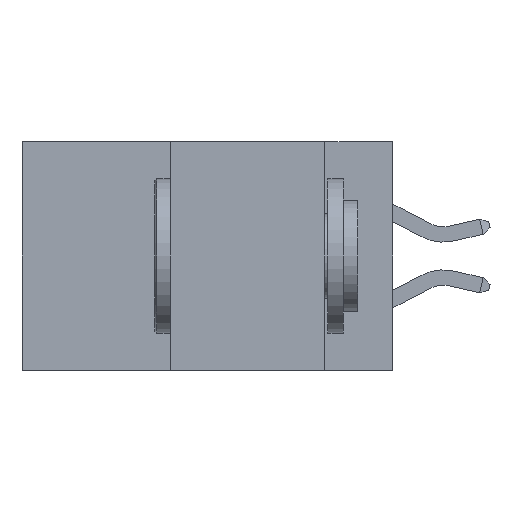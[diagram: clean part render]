
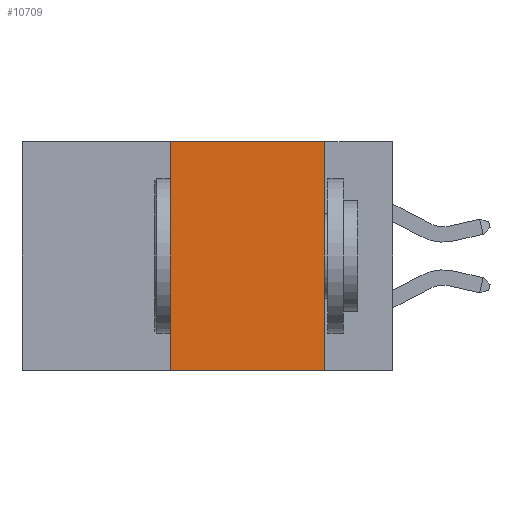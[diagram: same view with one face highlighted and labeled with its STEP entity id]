
A CAD part, left-side view. The second image highlights one B-rep face of the part: STEP entity #10709.
In plain terms, the highlighted planar face has unit normal (-1, 0, 0).
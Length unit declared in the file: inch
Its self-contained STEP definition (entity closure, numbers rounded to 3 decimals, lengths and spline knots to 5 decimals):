
#1151 = CARTESIAN_POINT ( 'NONE',  ( 0., 0.36, -0.37 ) ) ;
#1460 = VECTOR ( 'NONE', #2607, 39.37008 ) ;
#1481 = DIRECTION ( 'NONE',  ( 0., 0., -1. ) ) ;
#1838 = EDGE_CURVE ( 'NONE', #2828, #3553, #4318, .T. ) ;
#2607 = DIRECTION ( 'NONE',  ( 0., -1., 0. ) ) ;
#2828 = VERTEX_POINT ( 'NONE', #1151 ) ;
#3511 = VERTEX_POINT ( 'NONE', #5492 ) ;
#3553 = VERTEX_POINT ( 'NONE', #4721 ) ;
#4318 = LINE ( 'NONE', #9068, #7852 ) ;
#4686 = VECTOR ( 'NONE', #6363, 39.37008 ) ;
#4721 = CARTESIAN_POINT ( 'NONE',  ( 0., 0.36, 0. ) ) ;
#4734 = EDGE_CURVE ( 'NONE', #3553, #3511, #6600, .T. ) ;
#4755 = CARTESIAN_POINT ( 'NONE',  ( 0., 0.6, 0. ) ) ;
#4779 = DIRECTION ( 'NONE',  ( 0., -1., 0. ) ) ;
#5378 = CARTESIAN_POINT ( 'NONE',  ( 0., 0.11, 0. ) ) ;
#5492 = CARTESIAN_POINT ( 'NONE',  ( 0., 0.11, 0. ) ) ;
#5793 = AXIS2_PLACEMENT_3D ( 'NONE', #4755, #6771, #1481 ) ;
#6176 = FACE_OUTER_BOUND ( 'NONE', #7444, .T. ) ;
#6363 = DIRECTION ( 'NONE',  ( 0., 0., -1. ) ) ;
#6587 = PLANE ( 'NONE',  #5793 ) ;
#6600 = LINE ( 'NONE', #10134, #13108 ) ;
#6771 = DIRECTION ( 'NONE',  ( 1., 0., 0. ) ) ;
#7444 = EDGE_LOOP ( 'NONE', ( #9263, #10198, #8828, #8443 ) ) ;
#7852 = VECTOR ( 'NONE', #10008, 39.37008 ) ;
#8443 = ORIENTED_EDGE ( 'NONE', *, *, #11527, .T. ) ;
#8828 = ORIENTED_EDGE ( 'NONE', *, *, #1838, .F. ) ;
#9037 = CARTESIAN_POINT ( 'NONE',  ( 0., 0.6, -0.37 ) ) ;
#9068 = CARTESIAN_POINT ( 'NONE',  ( 0., 0.36, 0. ) ) ;
#9263 = ORIENTED_EDGE ( 'NONE', *, *, #9740, .F. ) ;
#9565 = CARTESIAN_POINT ( 'NONE',  ( 0., 0.11, -0.37 ) ) ;
#9740 = EDGE_CURVE ( 'NONE', #3511, #13769, #12524, .T. ) ;
#10008 = DIRECTION ( 'NONE',  ( 0., 0., 1. ) ) ;
#10134 = CARTESIAN_POINT ( 'NONE',  ( 0., 0.6, 0. ) ) ;
#10198 = ORIENTED_EDGE ( 'NONE', *, *, #4734, .F. ) ;
#10709 = ADVANCED_FACE ( 'NONE', ( #6176 ), #6587, .F. ) ;
#11527 = EDGE_CURVE ( 'NONE', #2828, #13769, #12148, .T. ) ;
#12148 = LINE ( 'NONE', #9037, #1460 ) ;
#12524 = LINE ( 'NONE', #5378, #4686 ) ;
#13108 = VECTOR ( 'NONE', #4779, 39.37008 ) ;
#13769 = VERTEX_POINT ( 'NONE', #9565 ) ;
